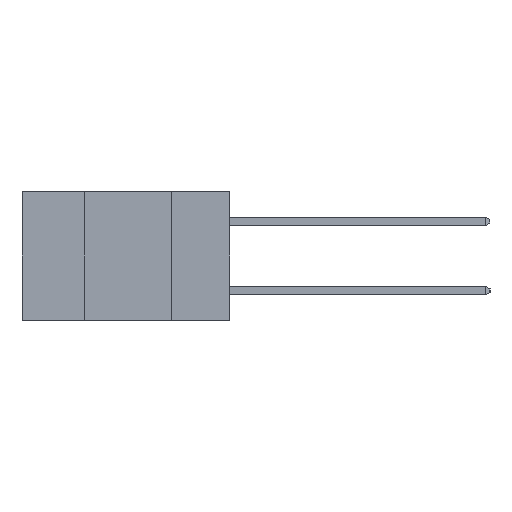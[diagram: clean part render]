
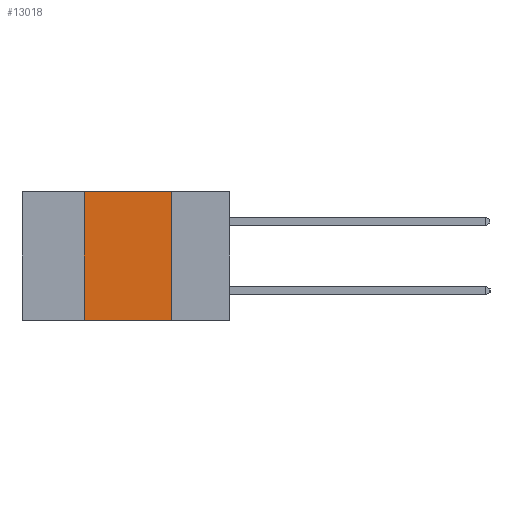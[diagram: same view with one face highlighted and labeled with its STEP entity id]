
A CAD part, left-side view. The second image highlights one B-rep face of the part: STEP entity #13018.
In plain terms, the highlighted planar face has unit normal (-1, 0, 0).
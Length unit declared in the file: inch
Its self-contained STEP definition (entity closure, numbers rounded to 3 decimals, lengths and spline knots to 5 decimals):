
#703 = LINE ( 'NONE', #7810, #11438 ) ;
#1055 = PLANE ( 'NONE',  #5133 ) ;
#1973 = CARTESIAN_POINT ( 'NONE',  ( 0., 0.42, -0.37 ) ) ;
#2607 = DIRECTION ( 'NONE',  ( 1., 0., 0. ) ) ;
#2653 = CARTESIAN_POINT ( 'NONE',  ( 0., 0.42, 0. ) ) ;
#2671 = LINE ( 'NONE', #4427, #14123 ) ;
#3425 = DIRECTION ( 'NONE',  ( 0., 0., -1. ) ) ;
#4427 = CARTESIAN_POINT ( 'NONE',  ( 0., 0.6, 0. ) ) ;
#5133 = AXIS2_PLACEMENT_3D ( 'NONE', #12616, #2607, #12685 ) ;
#5222 = ORIENTED_EDGE ( 'NONE', *, *, #15006, .F. ) ;
#5890 = DIRECTION ( 'NONE',  ( 0., -1., 0. ) ) ;
#6001 = DIRECTION ( 'NONE',  ( 0., -1., 0. ) ) ;
#6396 = ORIENTED_EDGE ( 'NONE', *, *, #16298, .F. ) ;
#7016 = LINE ( 'NONE', #12109, #17770 ) ;
#7701 = ORIENTED_EDGE ( 'NONE', *, *, #15589, .F. ) ;
#7810 = CARTESIAN_POINT ( 'NONE',  ( 0., 0.17, -0.37 ) ) ;
#8975 = EDGE_LOOP ( 'NONE', ( #7701, #5222, #6396, #13930 ) ) ;
#11438 = VECTOR ( 'NONE', #3425, 39.37008 ) ;
#11471 = CARTESIAN_POINT ( 'NONE',  ( 0., 0.17, -0.37 ) ) ;
#12109 = CARTESIAN_POINT ( 'NONE',  ( 0., 0.42, -0.37 ) ) ;
#12616 = CARTESIAN_POINT ( 'NONE',  ( 0., 0.6, 0. ) ) ;
#12685 = DIRECTION ( 'NONE',  ( 0., 0., -1. ) ) ;
#13018 = ADVANCED_FACE ( 'NONE', ( #17866 ), #1055, .F. ) ;
#13046 = CARTESIAN_POINT ( 'NONE',  ( 0., 0.6, -0.37 ) ) ;
#13540 = DIRECTION ( 'NONE',  ( 0., 0., 1. ) ) ;
#13770 = VERTEX_POINT ( 'NONE', #11471 ) ;
#13814 = CARTESIAN_POINT ( 'NONE',  ( 0., 0.17, 0. ) ) ;
#13930 = ORIENTED_EDGE ( 'NONE', *, *, #16054, .T. ) ;
#14123 = VECTOR ( 'NONE', #5890, 39.37008 ) ;
#14208 = VERTEX_POINT ( 'NONE', #13814 ) ;
#15006 = EDGE_CURVE ( 'NONE', #17115, #14208, #2671, .T. ) ;
#15589 = EDGE_CURVE ( 'NONE', #14208, #13770, #703, .T. ) ;
#16054 = EDGE_CURVE ( 'NONE', #17415, #13770, #18410, .T. ) ;
#16298 = EDGE_CURVE ( 'NONE', #17415, #17115, #7016, .T. ) ;
#17115 = VERTEX_POINT ( 'NONE', #2653 ) ;
#17415 = VERTEX_POINT ( 'NONE', #1973 ) ;
#17770 = VECTOR ( 'NONE', #13540, 39.37008 ) ;
#17866 = FACE_OUTER_BOUND ( 'NONE', #8975, .T. ) ;
#17985 = VECTOR ( 'NONE', #6001, 39.37008 ) ;
#18410 = LINE ( 'NONE', #13046, #17985 ) ;
